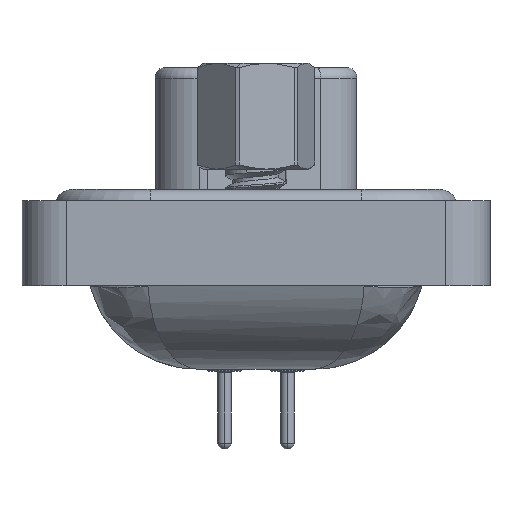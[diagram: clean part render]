
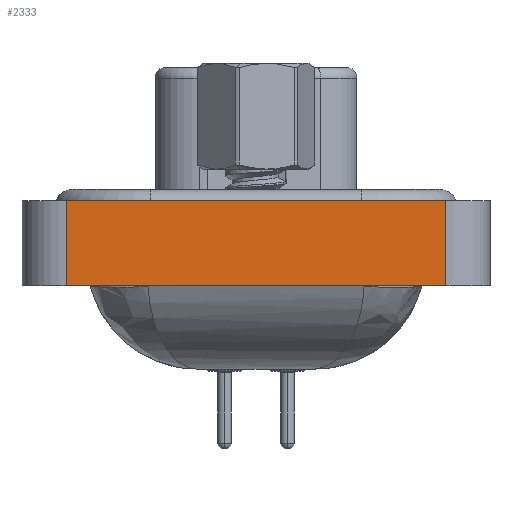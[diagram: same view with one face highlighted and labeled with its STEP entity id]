
A CAD part, left-side view. The second image highlights one B-rep face of the part: STEP entity #2333.
In plain terms, the highlighted planar face has unit normal (-1, 0, 0).
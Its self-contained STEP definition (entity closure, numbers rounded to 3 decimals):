
#190 = VECTOR ( 'NONE', #14001, 1000. ) ;
#451 = EDGE_CURVE ( 'NONE', #25419, #6068, #13447, .T. ) ;
#2333 = ADVANCED_FACE ( 'NONE', ( #6163 ), #6033, .T. ) ;
#3647 = ORIENTED_EDGE ( 'NONE', *, *, #26330, .T. ) ;
#3790 = DIRECTION ( 'NONE',  ( 0., 0., 1. ) ) ;
#3886 = CARTESIAN_POINT ( 'NONE',  ( -7.225, -8.55, -3.35 ) ) ;
#4632 = VECTOR ( 'NONE', #23440, 1000. ) ;
#5415 = CARTESIAN_POINT ( 'NONE',  ( -7.225, 8.55, -3.35 ) ) ;
#6033 = PLANE ( 'NONE',  #8984 ) ;
#6068 = VERTEX_POINT ( 'NONE', #15526 ) ;
#6163 = FACE_OUTER_BOUND ( 'NONE', #15534, .T. ) ;
#6637 = LINE ( 'NONE', #19491, #4632 ) ;
#7670 = LINE ( 'NONE', #20908, #190 ) ;
#7877 = ORIENTED_EDGE ( 'NONE', *, *, #451, .T. ) ;
#8984 = AXIS2_PLACEMENT_3D ( 'NONE', #16616, #25363, #3790 ) ;
#9237 = DIRECTION ( 'NONE',  ( 0., 0., 1. ) ) ;
#11807 = ORIENTED_EDGE ( 'NONE', *, *, #22447, .F. ) ;
#12260 = CARTESIAN_POINT ( 'NONE',  ( -7.225, 8.55, 0.5 ) ) ;
#12742 = VERTEX_POINT ( 'NONE', #12260 ) ;
#12918 = ORIENTED_EDGE ( 'NONE', *, *, #24053, .F. ) ;
#13447 = LINE ( 'NONE', #22063, #21500 ) ;
#14001 = DIRECTION ( 'NONE',  ( 0., -1., 0. ) ) ;
#15526 = CARTESIAN_POINT ( 'NONE',  ( -7.225, -8.55, 0.5 ) ) ;
#15534 = EDGE_LOOP ( 'NONE', ( #7877, #11807, #12918, #3647 ) ) ;
#16616 = CARTESIAN_POINT ( 'NONE',  ( -7.225, -8.55, -3.35 ) ) ;
#16904 = VECTOR ( 'NONE', #26719, 1000. ) ;
#18994 = CARTESIAN_POINT ( 'NONE',  ( -7.225, 8.55, -3.35 ) ) ;
#19491 = CARTESIAN_POINT ( 'NONE',  ( -7.225, -8.55, -3.35 ) ) ;
#20908 = CARTESIAN_POINT ( 'NONE',  ( -7.225, -8.55, 0.5 ) ) ;
#21500 = VECTOR ( 'NONE', #9237, 1000. ) ;
#22063 = CARTESIAN_POINT ( 'NONE',  ( -7.225, -8.55, -3.35 ) ) ;
#22165 = VERTEX_POINT ( 'NONE', #18994 ) ;
#22447 = EDGE_CURVE ( 'NONE', #12742, #6068, #7670, .T. ) ;
#23440 = DIRECTION ( 'NONE',  ( 0., -1., 0. ) ) ;
#24053 = EDGE_CURVE ( 'NONE', #22165, #12742, #24879, .T. ) ;
#24879 = LINE ( 'NONE', #5415, #16904 ) ;
#25363 = DIRECTION ( 'NONE',  ( -1., 0., 0. ) ) ;
#25419 = VERTEX_POINT ( 'NONE', #3886 ) ;
#26330 = EDGE_CURVE ( 'NONE', #22165, #25419, #6637, .T. ) ;
#26719 = DIRECTION ( 'NONE',  ( 0., 0., 1. ) ) ;
